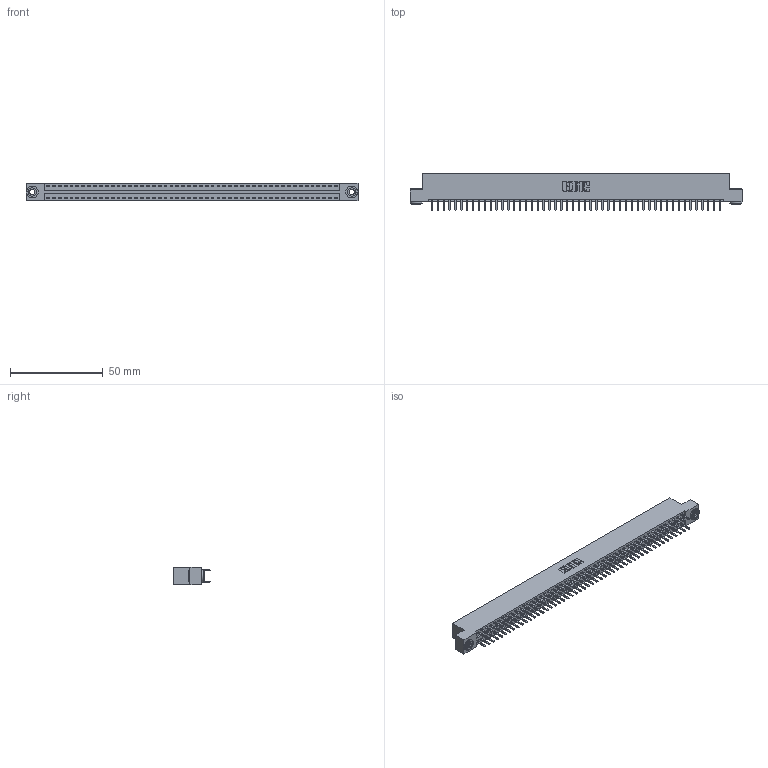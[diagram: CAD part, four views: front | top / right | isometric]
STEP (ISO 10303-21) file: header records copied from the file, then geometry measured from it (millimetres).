
FILE_DESCRIPTION (( 'STEP AP203' ), '1' );
FILE_NAME ('346-100-520-203.STEP', '2018-08-30T10:10:44', ( '' ), ( '' ), 'SwSTEP 2.0', 'SolidWorks 2016', '' );
FILE_SCHEMA (( 'CONFIG_CONTROL_DESIGN' ));
Length unit declared in the file: inch
Products named in the file (4): 346 Part_Flush Mounting Lugs - 0.156 Dia-TH; 345-292-001_345-293-120; 345-250-002_345-250-002-102; 346-100-520-203
Assembly tree (103 placements, depth 2):
  346-100-520-203
    346 Part_Flush Mounting Lugs - 0.156 Dia-TH
    345-292-001_345-293-120  x100
    345-250-002_345-250-002-102  x2
Bounding box: 179.32 x 20.02 x 9.4 mm (x, y, z)
Volume: 17523.9 mm3; surface area: 24324.7 mm2
Topology: 103 solids, 103 shells, 5760 faces, 16705 edges, 10866 vertices
Faces by surface type: plane 3786, cylinder 1966, cone 8
Entity records: 32318 total; most frequent: CARTESIAN_POINT 5303, ORIENTED_EDGE 5218, DIRECTION 4743, EDGE_CURVE 2609, VECTOR 2249, LINE 2249, VERTEX_POINT 1734, AXIS2_PLACEMENT_3D 1247
